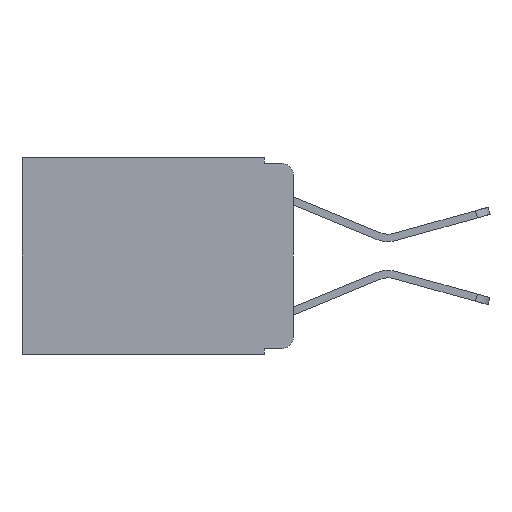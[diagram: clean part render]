
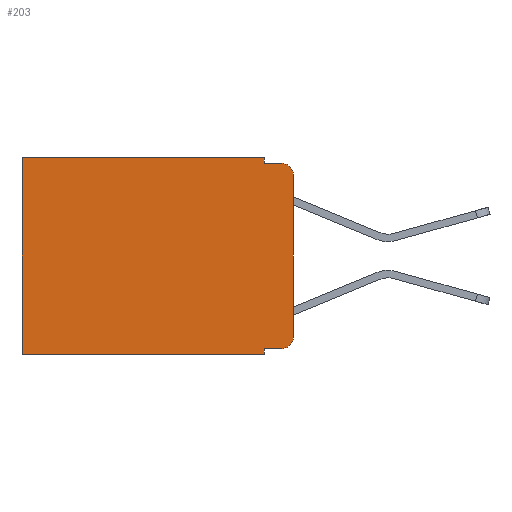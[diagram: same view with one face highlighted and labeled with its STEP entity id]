
A CAD part, left-side view. The second image highlights one B-rep face of the part: STEP entity #203.
In plain terms, the highlighted planar face has unit normal (-1, 0, 0).
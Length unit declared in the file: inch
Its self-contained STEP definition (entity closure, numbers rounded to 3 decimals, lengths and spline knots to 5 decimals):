
#203 = ADVANCED_FACE ( 'NONE', ( #8020 ), #8309, .F. ) ;
#230 = EDGE_CURVE ( 'NONE', #2381, #4419, #7675, .T. ) ;
#287 = VERTEX_POINT ( 'NONE', #948 ) ;
#658 = VERTEX_POINT ( 'NONE', #6065 ) ;
#948 = CARTESIAN_POINT ( 'NONE',  ( 0.298, 0.02, -0.333 ) ) ;
#1084 = EDGE_CURVE ( 'NONE', #2381, #287, #1538, .T. ) ;
#1159 = EDGE_CURVE ( 'NONE', #4419, #7860, #6913, .T. ) ;
#1185 = CARTESIAN_POINT ( 'NONE',  ( 0.298, 0., 0. ) ) ;
#1224 = VECTOR ( 'NONE', #3306, 39.37008 ) ;
#1330 = CARTESIAN_POINT ( 'NONE',  ( 0.298, 0.02, -0.313 ) ) ;
#1422 = EDGE_CURVE ( 'NONE', #5852, #1765, #3963, .T. ) ;
#1512 = CARTESIAN_POINT ( 'NONE',  ( 0.298, 0., -0.03 ) ) ;
#1538 = LINE ( 'NONE', #6731, #3258 ) ;
#1765 = VERTEX_POINT ( 'NONE', #2664 ) ;
#1927 = DIRECTION ( 'NONE',  ( 0., 0., -1. ) ) ;
#2196 = VECTOR ( 'NONE', #2383, 39.37008 ) ;
#2263 = DIRECTION ( 'NONE',  ( 0., 1., 0. ) ) ;
#2341 = CARTESIAN_POINT ( 'NONE',  ( 0.298, 0.473, 0. ) ) ;
#2356 = VECTOR ( 'NONE', #2263, 39.37008 ) ;
#2381 = VERTEX_POINT ( 'NONE', #4761 ) ;
#2383 = DIRECTION ( 'NONE',  ( 0., 0., -1. ) ) ;
#2635 = EDGE_CURVE ( 'NONE', #5987, #1765, #7081, .T. ) ;
#2664 = CARTESIAN_POINT ( 'NONE',  ( 0.298, 0.02, -0.01 ) ) ;
#2772 = EDGE_CURVE ( 'NONE', #5852, #5804, #7904, .T. ) ;
#2884 = CIRCLE ( 'NONE', #7607, 0.02 ) ;
#2904 = CARTESIAN_POINT ( 'NONE',  ( 0.298, 0., -0.313 ) ) ;
#3011 = VERTEX_POINT ( 'NONE', #5019 ) ;
#3076 = EDGE_CURVE ( 'NONE', #287, #5804, #2884, .T. ) ;
#3258 = VECTOR ( 'NONE', #5041, 39.37008 ) ;
#3306 = DIRECTION ( 'NONE',  ( 0., -1., 0. ) ) ;
#3817 = DIRECTION ( 'NONE',  ( 1., 0., 0. ) ) ;
#3883 = LINE ( 'NONE', #5485, #7150 ) ;
#3963 = CIRCLE ( 'NONE', #5384, 0.02 ) ;
#4272 = CARTESIAN_POINT ( 'NONE',  ( 0.298, 0.02, -0.03 ) ) ;
#4419 = VERTEX_POINT ( 'NONE', #5303 ) ;
#4565 = ORIENTED_EDGE ( 'NONE', *, *, #1422, .T. ) ;
#4583 = ORIENTED_EDGE ( 'NONE', *, *, #2635, .F. ) ;
#4641 = ORIENTED_EDGE ( 'NONE', *, *, #2772, .F. ) ;
#4702 = ORIENTED_EDGE ( 'NONE', *, *, #4856, .F. ) ;
#4722 = ORIENTED_EDGE ( 'NONE', *, *, #1084, .T. ) ;
#4749 = ORIENTED_EDGE ( 'NONE', *, *, #230, .F. ) ;
#4750 = ORIENTED_EDGE ( 'NONE', *, *, #3076, .T. ) ;
#4761 = CARTESIAN_POINT ( 'NONE',  ( 0.298, 0.051, -0.333 ) ) ;
#4779 = ORIENTED_EDGE ( 'NONE', *, *, #8148, .T. ) ;
#4795 = ORIENTED_EDGE ( 'NONE', *, *, #6769, .T. ) ;
#4830 = ORIENTED_EDGE ( 'NONE', *, *, #1159, .F. ) ;
#4856 = EDGE_CURVE ( 'NONE', #658, #5987, #3883, .T. ) ;
#5019 = CARTESIAN_POINT ( 'NONE',  ( 0.298, 0.473, 0. ) ) ;
#5041 = DIRECTION ( 'NONE',  ( 0., -1., 0. ) ) ;
#5084 = VECTOR ( 'NONE', #7576, 39.37008 ) ;
#5108 = CARTESIAN_POINT ( 'NONE',  ( 0.298, 0.051, 0. ) ) ;
#5303 = CARTESIAN_POINT ( 'NONE',  ( 0.298, 0.051, -0.343 ) ) ;
#5330 = CARTESIAN_POINT ( 'NONE',  ( 0.298, 0.051, -0.01 ) ) ;
#5384 = AXIS2_PLACEMENT_3D ( 'NONE', #4272, #8847, #8822 ) ;
#5485 = CARTESIAN_POINT ( 'NONE',  ( 0.298, 0.051, 0. ) ) ;
#5790 = CARTESIAN_POINT ( 'NONE',  ( 0.298, 0.473, -0.343 ) ) ;
#5804 = VERTEX_POINT ( 'NONE', #2904 ) ;
#5852 = VERTEX_POINT ( 'NONE', #1512 ) ;
#5987 = VERTEX_POINT ( 'NONE', #6447 ) ;
#6065 = CARTESIAN_POINT ( 'NONE',  ( 0.298, 0.051, 0. ) ) ;
#6258 = DIRECTION ( 'NONE',  ( 0., 0., -1. ) ) ;
#6288 = VECTOR ( 'NONE', #1927, 39.37008 ) ;
#6291 = AXIS2_PLACEMENT_3D ( 'NONE', #8313, #3817, #7088 ) ;
#6447 = CARTESIAN_POINT ( 'NONE',  ( 0.298, 0.051, -0.01 ) ) ;
#6731 = CARTESIAN_POINT ( 'NONE',  ( 0.298, 0.051, -0.333 ) ) ;
#6769 = EDGE_CURVE ( 'NONE', #658, #3011, #7965, .T. ) ;
#6913 = LINE ( 'NONE', #8063, #5084 ) ;
#7042 = DIRECTION ( 'NONE',  ( -1., 0., 0. ) ) ;
#7081 = LINE ( 'NONE', #5330, #1224 ) ;
#7088 = DIRECTION ( 'NONE',  ( 0., 0., -1. ) ) ;
#7150 = VECTOR ( 'NONE', #8689, 39.37008 ) ;
#7165 = LINE ( 'NONE', #2341, #8530 ) ;
#7214 = EDGE_LOOP ( 'NONE', ( #4641, #4565, #4583, #4702, #4795, #4779, #4830, #4749, #4722, #4750 ) ) ;
#7300 = CARTESIAN_POINT ( 'NONE',  ( 0.298, 0., 0. ) ) ;
#7576 = DIRECTION ( 'NONE',  ( 0., 1., 0. ) ) ;
#7607 = AXIS2_PLACEMENT_3D ( 'NONE', #1330, #7042, #6258 ) ;
#7675 = LINE ( 'NONE', #5108, #2196 ) ;
#7823 = DIRECTION ( 'NONE',  ( 0., 0., -1. ) ) ;
#7860 = VERTEX_POINT ( 'NONE', #5790 ) ;
#7904 = LINE ( 'NONE', #7300, #6288 ) ;
#7965 = LINE ( 'NONE', #1185, #2356 ) ;
#8020 = FACE_OUTER_BOUND ( 'NONE', #7214, .T. ) ;
#8063 = CARTESIAN_POINT ( 'NONE',  ( 0.298, 0., -0.343 ) ) ;
#8148 = EDGE_CURVE ( 'NONE', #3011, #7860, #7165, .T. ) ;
#8309 = PLANE ( 'NONE',  #6291 ) ;
#8313 = CARTESIAN_POINT ( 'NONE',  ( 0.298, 0., 0. ) ) ;
#8530 = VECTOR ( 'NONE', #7823, 39.37008 ) ;
#8689 = DIRECTION ( 'NONE',  ( 0., 0., -1. ) ) ;
#8822 = DIRECTION ( 'NONE',  ( 0., 0., -1. ) ) ;
#8847 = DIRECTION ( 'NONE',  ( -1., 0., 0. ) ) ;
